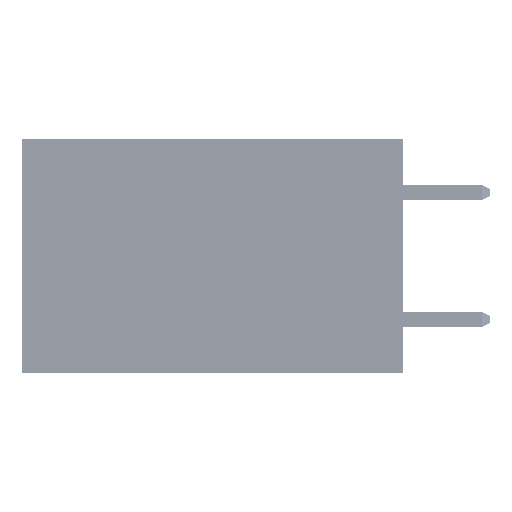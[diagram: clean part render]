
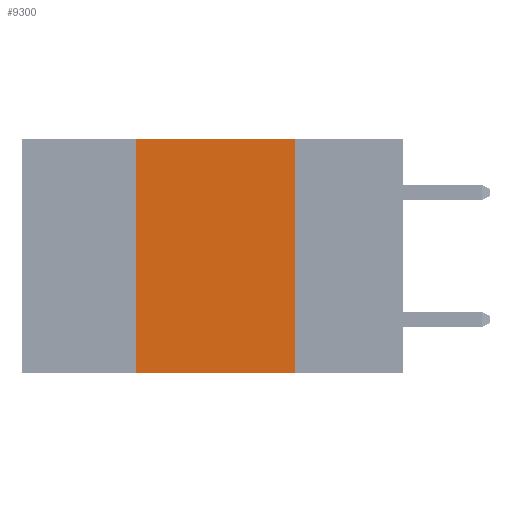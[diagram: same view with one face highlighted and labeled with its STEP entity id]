
A CAD part, left-side view. The second image highlights one B-rep face of the part: STEP entity #9300.
In plain terms, the highlighted planar face has unit normal (-1, 0, 0).
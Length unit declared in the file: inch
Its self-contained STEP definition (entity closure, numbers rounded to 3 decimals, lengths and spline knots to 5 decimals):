
#863 = VERTEX_POINT ( 'NONE', #45950 ) ;
#1494 = DIRECTION ( 'NONE',  ( 0., 0., -1. ) ) ;
#4007 = CARTESIAN_POINT ( 'NONE',  ( 0., 0.6, 0. ) ) ;
#5567 = CARTESIAN_POINT ( 'NONE',  ( 0., 0.17, 0. ) ) ;
#5807 = LINE ( 'NONE', #12053, #25878 ) ;
#8645 = CARTESIAN_POINT ( 'NONE',  ( 0., 0.42, -0.37 ) ) ;
#9300 = ADVANCED_FACE ( 'NONE', ( #10737 ), #22534, .F. ) ;
#10428 = CARTESIAN_POINT ( 'NONE',  ( 0., 0.42, 0. ) ) ;
#10638 = DIRECTION ( 'NONE',  ( 1., 0., 0. ) ) ;
#10737 = FACE_OUTER_BOUND ( 'NONE', #49038, .T. ) ;
#12053 = CARTESIAN_POINT ( 'NONE',  ( 0., 0.42, 0. ) ) ;
#13442 = AXIS2_PLACEMENT_3D ( 'NONE', #50537, #10638, #38638 ) ;
#16061 = DIRECTION ( 'NONE',  ( 0., 0., 1. ) ) ;
#16757 = ORIENTED_EDGE ( 'NONE', *, *, #26388, .T. ) ;
#18032 = VECTOR ( 'NONE', #28044, 39.37008 ) ;
#21871 = VECTOR ( 'NONE', #1494, 39.37008 ) ;
#22534 = PLANE ( 'NONE',  #13442 ) ;
#23121 = LINE ( 'NONE', #5567, #21871 ) ;
#25565 = ORIENTED_EDGE ( 'NONE', *, *, #50606, .F. ) ;
#25804 = VECTOR ( 'NONE', #35722, 39.37008 ) ;
#25878 = VECTOR ( 'NONE', #16061, 39.37008 ) ;
#26388 = EDGE_CURVE ( 'NONE', #34493, #29225, #48372, .T. ) ;
#28044 = DIRECTION ( 'NONE',  ( 0., -1., 0. ) ) ;
#29225 = VERTEX_POINT ( 'NONE', #36687 ) ;
#29330 = ORIENTED_EDGE ( 'NONE', *, *, #30573, .F. ) ;
#30573 = EDGE_CURVE ( 'NONE', #863, #29225, #23121, .T. ) ;
#31183 = ORIENTED_EDGE ( 'NONE', *, *, #47169, .F. ) ;
#31704 = CARTESIAN_POINT ( 'NONE',  ( 0., 0.6, -0.37 ) ) ;
#32192 = VERTEX_POINT ( 'NONE', #10428 ) ;
#34493 = VERTEX_POINT ( 'NONE', #8645 ) ;
#35722 = DIRECTION ( 'NONE',  ( 0., -1., 0. ) ) ;
#36687 = CARTESIAN_POINT ( 'NONE',  ( 0., 0.17, -0.37 ) ) ;
#38638 = DIRECTION ( 'NONE',  ( 0., 0., -1. ) ) ;
#45950 = CARTESIAN_POINT ( 'NONE',  ( 0., 0.17, 0. ) ) ;
#47169 = EDGE_CURVE ( 'NONE', #34493, #32192, #5807, .T. ) ;
#48372 = LINE ( 'NONE', #31704, #25804 ) ;
#49038 = EDGE_LOOP ( 'NONE', ( #29330, #25565, #31183, #16757 ) ) ;
#50001 = LINE ( 'NONE', #4007, #18032 ) ;
#50537 = CARTESIAN_POINT ( 'NONE',  ( 0., 0.6, 0. ) ) ;
#50606 = EDGE_CURVE ( 'NONE', #32192, #863, #50001, .T. ) ;
